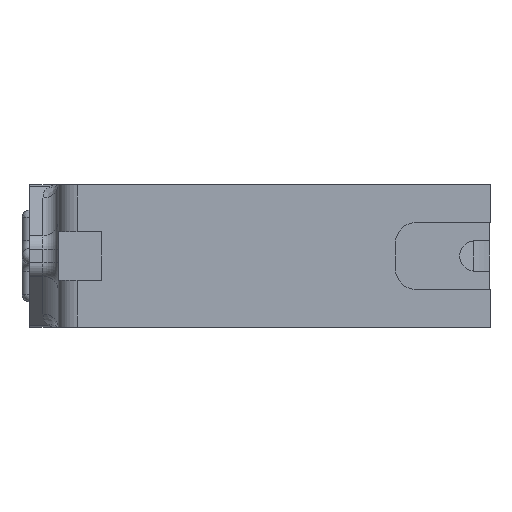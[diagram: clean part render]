
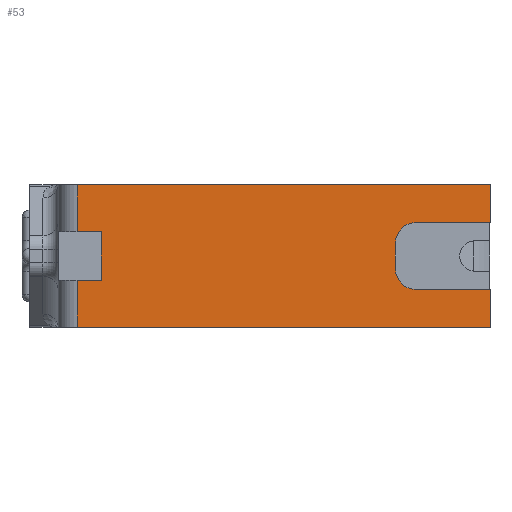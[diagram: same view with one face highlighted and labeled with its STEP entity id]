
A CAD part, left-side view. The second image highlights one B-rep face of the part: STEP entity #53.
In plain terms, the highlighted planar face has unit normal (-1, 0, 0).
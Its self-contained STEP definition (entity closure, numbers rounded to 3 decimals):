
#53 = ADVANCED_FACE ( 'NONE', ( #2998 ), #7407, .T. ) ;
#140 = CARTESIAN_POINT ( 'NONE',  ( 0.291, -254.19, 23.114 ) ) ;
#163 = DIRECTION ( 'NONE',  ( -1., 0., 0. ) ) ;
#337 = LINE ( 'NONE', #6164, #6426 ) ;
#451 = VERTEX_POINT ( 'NONE', #7502 ) ;
#477 = CARTESIAN_POINT ( 'NONE',  ( 0.291, -342.677, -4.216 ) ) ;
#585 = CARTESIAN_POINT ( 'NONE',  ( 0.291, -254.19, -4.216 ) ) ;
#620 = LINE ( 'NONE', #2783, #6873 ) ;
#995 = ORIENTED_EDGE ( 'NONE', *, *, #4517, .T. ) ;
#1040 = CARTESIAN_POINT ( 'NONE',  ( 0.291, -342.677, 13.31 ) ) ;
#1045 = DIRECTION ( 'NONE',  ( 0., 0., -1. ) ) ;
#1076 = DIRECTION ( 'NONE',  ( 0., -1., 0. ) ) ;
#1115 = LINE ( 'NONE', #1469, #1306 ) ;
#1205 = AXIS2_PLACEMENT_3D ( 'NONE', #6548, #3024, #7132 ) ;
#1270 = DIRECTION ( 'NONE',  ( 0., 0., -1. ) ) ;
#1306 = VECTOR ( 'NONE', #4582, 1000. ) ;
#1394 = CARTESIAN_POINT ( 'NONE',  ( 0.291, -254.19, 23.114 ) ) ;
#1408 = VERTEX_POINT ( 'NONE', #1040 ) ;
#1431 = VERTEX_POINT ( 'NONE', #7634 ) ;
#1449 = ORIENTED_EDGE ( 'NONE', *, *, #6458, .T. ) ;
#1469 = CARTESIAN_POINT ( 'NONE',  ( 0.291, -254.19, -9.74 ) ) ;
#1581 = ORIENTED_EDGE ( 'NONE', *, *, #1809, .T. ) ;
#1615 = EDGE_CURVE ( 'NONE', #1431, #7532, #6844, .T. ) ;
#1674 = VECTOR ( 'NONE', #3094, 1000. ) ;
#1809 = EDGE_CURVE ( 'NONE', #6839, #7371, #2978, .T. ) ;
#1968 = EDGE_CURVE ( 'NONE', #4667, #6810, #7286, .T. ) ;
#2005 = EDGE_CURVE ( 'NONE', #5287, #1408, #5573, .T. ) ;
#2030 = DIRECTION ( 'NONE',  ( 0., 1., 0. ) ) ;
#2093 = VECTOR ( 'NONE', #1045, 1000. ) ;
#2154 = CARTESIAN_POINT ( 'NONE',  ( 0.291, -361.831, -4.216 ) ) ;
#2210 = CIRCLE ( 'NONE', #4884, 5.556 ) ;
#2234 = CARTESIAN_POINT ( 'NONE',  ( 0.291, -361.831, -9.74 ) ) ;
#2271 = ORIENTED_EDGE ( 'NONE', *, *, #7417, .T. ) ;
#2310 = CARTESIAN_POINT ( 'NONE',  ( 0.291, -337.121, 1.341 ) ) ;
#2356 = CARTESIAN_POINT ( 'NONE',  ( 0.291, -254.19, -14.019 ) ) ;
#2386 = VECTOR ( 'NONE', #1076, 1000. ) ;
#2430 = AXIS2_PLACEMENT_3D ( 'NONE', #2684, #163, #4521 ) ;
#2484 = ORIENTED_EDGE ( 'NONE', *, *, #6482, .T. ) ;
#2684 = CARTESIAN_POINT ( 'NONE',  ( 0.291, -254.19, -9.74 ) ) ;
#2690 = EDGE_LOOP ( 'NONE', ( #4549, #2271, #3787, #7346, #2484, #2731, #1581, #995, #1449, #3469, #4545, #3348, #4777, #7263 ) ) ;
#2696 = CARTESIAN_POINT ( 'NONE',  ( 0.291, -254.19, 10.897 ) ) ;
#2731 = ORIENTED_EDGE ( 'NONE', *, *, #6149, .T. ) ;
#2783 = CARTESIAN_POINT ( 'NONE',  ( 0.291, -337.121, -9.74 ) ) ;
#2875 = DIRECTION ( 'NONE',  ( 0., 0., 1. ) ) ;
#2974 = DIRECTION ( 'NONE',  ( 1., 0., 0. ) ) ;
#2978 = LINE ( 'NONE', #5325, #1674 ) ;
#2998 = FACE_OUTER_BOUND ( 'NONE', #2690, .T. ) ;
#3024 = DIRECTION ( 'NONE',  ( 1., 0., 0. ) ) ;
#3085 = EDGE_CURVE ( 'NONE', #5632, #1431, #5388, .T. ) ;
#3094 = DIRECTION ( 'NONE',  ( 0., -1., 0. ) ) ;
#3115 = DIRECTION ( 'NONE',  ( 0., 1., 0. ) ) ;
#3131 = EDGE_CURVE ( 'NONE', #1408, #5632, #6924, .T. ) ;
#3267 = CARTESIAN_POINT ( 'NONE',  ( 0.291, -260.54, -1.803 ) ) ;
#3348 = ORIENTED_EDGE ( 'NONE', *, *, #2005, .T. ) ;
#3384 = LINE ( 'NONE', #4740, #2093 ) ;
#3469 = ORIENTED_EDGE ( 'NONE', *, *, #6314, .T. ) ;
#3621 = CARTESIAN_POINT ( 'NONE',  ( 0.291, -254.19, 10.897 ) ) ;
#3650 = VECTOR ( 'NONE', #7579, 1000. ) ;
#3733 = CARTESIAN_POINT ( 'NONE',  ( 0.291, -254.19, -1.803 ) ) ;
#3757 = VECTOR ( 'NONE', #2030, 1000. ) ;
#3787 = ORIENTED_EDGE ( 'NONE', *, *, #1968, .T. ) ;
#3808 = VERTEX_POINT ( 'NONE', #2310 ) ;
#3873 = DIRECTION ( 'NONE',  ( 0., 0., 1. ) ) ;
#4079 = VERTEX_POINT ( 'NONE', #2154 ) ;
#4110 = CARTESIAN_POINT ( 'NONE',  ( 0.291, -254.19, 13.31 ) ) ;
#4161 = CARTESIAN_POINT ( 'NONE',  ( 0.291, -260.54, 10.897 ) ) ;
#4208 = VECTOR ( 'NONE', #2875, 1000. ) ;
#4517 = EDGE_CURVE ( 'NONE', #7371, #4079, #337, .T. ) ;
#4521 = DIRECTION ( 'NONE',  ( 0., -1., 0. ) ) ;
#4545 = ORIENTED_EDGE ( 'NONE', *, *, #5793, .T. ) ;
#4549 = ORIENTED_EDGE ( 'NONE', *, *, #1615, .T. ) ;
#4582 = DIRECTION ( 'NONE',  ( 0., 0., -1. ) ) ;
#4614 = DIRECTION ( 'NONE',  ( 0., 0., 1. ) ) ;
#4667 = VERTEX_POINT ( 'NONE', #2696 ) ;
#4683 = VECTOR ( 'NONE', #1270, 1000. ) ;
#4690 = LINE ( 'NONE', #585, #6414 ) ;
#4740 = CARTESIAN_POINT ( 'NONE',  ( 0.291, -260.54, -9.74 ) ) ;
#4777 = ORIENTED_EDGE ( 'NONE', *, *, #3131, .T. ) ;
#4874 = LINE ( 'NONE', #3733, #6061 ) ;
#4884 = AXIS2_PLACEMENT_3D ( 'NONE', #6504, #2974, #7089 ) ;
#4905 = DIRECTION ( 'NONE',  ( 0., 1., 0. ) ) ;
#4956 = CARTESIAN_POINT ( 'NONE',  ( 0.291, -361.831, -14.019 ) ) ;
#5287 = VERTEX_POINT ( 'NONE', #5669 ) ;
#5325 = CARTESIAN_POINT ( 'NONE',  ( 0.291, -254.19, -14.019 ) ) ;
#5388 = LINE ( 'NONE', #2234, #4208 ) ;
#5554 = CARTESIAN_POINT ( 'NONE',  ( 0.291, -361.831, 13.31 ) ) ;
#5573 = CIRCLE ( 'NONE', #1205, 5.556 ) ;
#5632 = VERTEX_POINT ( 'NONE', #5554 ) ;
#5669 = CARTESIAN_POINT ( 'NONE',  ( 0.291, -337.121, 7.754 ) ) ;
#5793 = EDGE_CURVE ( 'NONE', #3808, #5287, #620, .T. ) ;
#6014 = VERTEX_POINT ( 'NONE', #477 ) ;
#6061 = VECTOR ( 'NONE', #3115, 1000. ) ;
#6149 = EDGE_CURVE ( 'NONE', #451, #6839, #1115, .T. ) ;
#6164 = CARTESIAN_POINT ( 'NONE',  ( 0.291, -361.831, -9.74 ) ) ;
#6314 = EDGE_CURVE ( 'NONE', #6014, #3808, #2210, .T. ) ;
#6414 = VECTOR ( 'NONE', #4905, 1000. ) ;
#6426 = VECTOR ( 'NONE', #3873, 1000. ) ;
#6458 = EDGE_CURVE ( 'NONE', #4079, #6014, #4690, .T. ) ;
#6482 = EDGE_CURVE ( 'NONE', #7010, #451, #4874, .T. ) ;
#6504 = CARTESIAN_POINT ( 'NONE',  ( 0.291, -342.677, 1.341 ) ) ;
#6548 = CARTESIAN_POINT ( 'NONE',  ( 0.291, -342.677, 7.754 ) ) ;
#6810 = VERTEX_POINT ( 'NONE', #4161 ) ;
#6839 = VERTEX_POINT ( 'NONE', #2356 ) ;
#6844 = LINE ( 'NONE', #1394, #3757 ) ;
#6873 = VECTOR ( 'NONE', #4614, 1000. ) ;
#6924 = LINE ( 'NONE', #4110, #3650 ) ;
#7010 = VERTEX_POINT ( 'NONE', #3267 ) ;
#7089 = DIRECTION ( 'NONE',  ( 0., -1., 0. ) ) ;
#7132 = DIRECTION ( 'NONE',  ( 0., 1., 0. ) ) ;
#7263 = ORIENTED_EDGE ( 'NONE', *, *, #3085, .T. ) ;
#7280 = CARTESIAN_POINT ( 'NONE',  ( 0.291, -254.19, -9.74 ) ) ;
#7286 = LINE ( 'NONE', #3621, #2386 ) ;
#7346 = ORIENTED_EDGE ( 'NONE', *, *, #7753, .T. ) ;
#7371 = VERTEX_POINT ( 'NONE', #4956 ) ;
#7407 = PLANE ( 'NONE',  #2430 ) ;
#7417 = EDGE_CURVE ( 'NONE', #7532, #4667, #7769, .T. ) ;
#7502 = CARTESIAN_POINT ( 'NONE',  ( 0.291, -254.19, -1.803 ) ) ;
#7532 = VERTEX_POINT ( 'NONE', #140 ) ;
#7579 = DIRECTION ( 'NONE',  ( 0., -1., 0. ) ) ;
#7634 = CARTESIAN_POINT ( 'NONE',  ( 0.291, -361.831, 23.114 ) ) ;
#7753 = EDGE_CURVE ( 'NONE', #6810, #7010, #3384, .T. ) ;
#7769 = LINE ( 'NONE', #7280, #4683 ) ;
